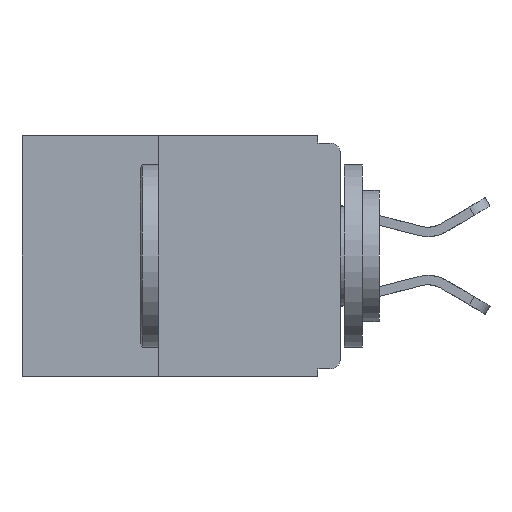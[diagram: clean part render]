
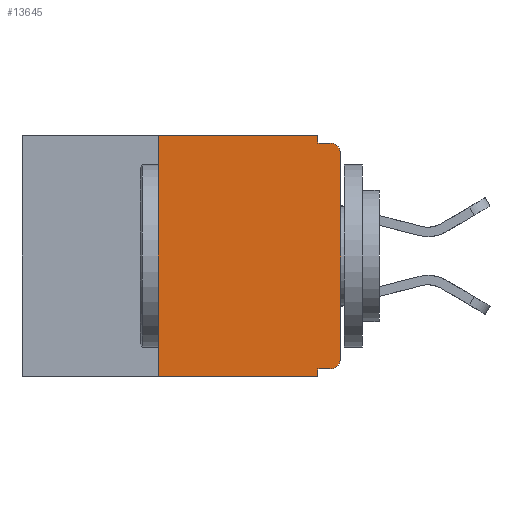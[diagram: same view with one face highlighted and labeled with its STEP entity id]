
A CAD part, left-side view. The second image highlights one B-rep face of the part: STEP entity #13645.
In plain terms, the highlighted planar face has unit normal (-1, 0, 0).
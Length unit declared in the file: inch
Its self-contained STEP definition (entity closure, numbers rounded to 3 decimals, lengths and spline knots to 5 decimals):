
#444 = EDGE_CURVE ( 'NONE', #15665, #19571, #15743, .T. ) ;
#541 = EDGE_CURVE ( 'NONE', #19571, #7961, #1320, .T. ) ;
#858 = CARTESIAN_POINT ( 'NONE',  ( 0., 0., 0. ) ) ;
#886 = LINE ( 'NONE', #4013, #8792 ) ;
#1320 = LINE ( 'NONE', #17184, #17396 ) ;
#1371 = ORIENTED_EDGE ( 'NONE', *, *, #14085, .F. ) ;
#1506 = VECTOR ( 'NONE', #18126, 39.37008 ) ;
#1526 = ORIENTED_EDGE ( 'NONE', *, *, #541, .F. ) ;
#1555 = DIRECTION ( 'NONE',  ( 0., 0., -1. ) ) ;
#1747 = ORIENTED_EDGE ( 'NONE', *, *, #4567, .T. ) ;
#1749 = ORIENTED_EDGE ( 'NONE', *, *, #18401, .T. ) ;
#2271 = DIRECTION ( 'NONE',  ( -1., 0., 0. ) ) ;
#2449 = DIRECTION ( 'NONE',  ( 0., 0., -1. ) ) ;
#2571 = ORIENTED_EDGE ( 'NONE', *, *, #444, .F. ) ;
#3269 = CARTESIAN_POINT ( 'NONE',  ( 0., 0.031, 0. ) ) ;
#3664 = ORIENTED_EDGE ( 'NONE', *, *, #14393, .F. ) ;
#4013 = CARTESIAN_POINT ( 'NONE',  ( 0., 0.031, -0.33 ) ) ;
#4156 = EDGE_CURVE ( 'NONE', #10617, #11605, #9327, .T. ) ;
#4250 = DIRECTION ( 'NONE',  ( 0., -1., 0. ) ) ;
#4461 = VECTOR ( 'NONE', #12520, 39.37008 ) ;
#4567 = EDGE_CURVE ( 'NONE', #10539, #11439, #19518, .T. ) ;
#4672 = CARTESIAN_POINT ( 'NONE',  ( 0., 0.437, 0. ) ) ;
#4849 = DIRECTION ( 'NONE',  ( 0., 1., 0. ) ) ;
#5137 = VECTOR ( 'NONE', #11499, 39.37008 ) ;
#5409 = VECTOR ( 'NONE', #5617, 39.37008 ) ;
#5617 = DIRECTION ( 'NONE',  ( 0., 0., 1. ) ) ;
#5686 = CARTESIAN_POINT ( 'NONE',  ( 0., 0.437, 0. ) ) ;
#6253 = PLANE ( 'NONE',  #17748 ) ;
#6375 = CARTESIAN_POINT ( 'NONE',  ( 0., 0.015, -0.32 ) ) ;
#6379 = ORIENTED_EDGE ( 'NONE', *, *, #7638, .T. ) ;
#6568 = CARTESIAN_POINT ( 'NONE',  ( 0., 0.25, -0.33 ) ) ;
#6708 = CARTESIAN_POINT ( 'NONE',  ( 0., 0.031, -0.33 ) ) ;
#6835 = EDGE_CURVE ( 'NONE', #10617, #7065, #15927, .T. ) ;
#6854 = ORIENTED_EDGE ( 'NONE', *, *, #4156, .F. ) ;
#6856 = EDGE_LOOP ( 'NONE', ( #6379, #1749, #1526, #2571, #1371, #6854, #17274, #17053, #3664, #1747 ) ) ;
#7065 = VERTEX_POINT ( 'NONE', #6708 ) ;
#7445 = CARTESIAN_POINT ( 'NONE',  ( 0., 0.25, 0. ) ) ;
#7638 = EDGE_CURVE ( 'NONE', #11439, #8525, #9589, .T. ) ;
#7961 = VERTEX_POINT ( 'NONE', #15674 ) ;
#8308 = VERTEX_POINT ( 'NONE', #17842 ) ;
#8525 = VERTEX_POINT ( 'NONE', #12263 ) ;
#8621 = CARTESIAN_POINT ( 'NONE',  ( 0., 0., -0.305 ) ) ;
#8653 = VECTOR ( 'NONE', #4849, 39.37008 ) ;
#8792 = VECTOR ( 'NONE', #2449, 39.37008 ) ;
#9327 = LINE ( 'NONE', #11340, #5137 ) ;
#9476 = EDGE_CURVE ( 'NONE', #8308, #7065, #886, .T. ) ;
#9589 = LINE ( 'NONE', #858, #5409 ) ;
#9760 = DIRECTION ( 'NONE',  ( 0., 0., -1. ) ) ;
#10539 = VERTEX_POINT ( 'NONE', #6375 ) ;
#10617 = VERTEX_POINT ( 'NONE', #6568 ) ;
#10971 = DIRECTION ( 'NONE',  ( 1., 0., 0. ) ) ;
#11340 = CARTESIAN_POINT ( 'NONE',  ( 0., 0.25, -0.33 ) ) ;
#11436 = CARTESIAN_POINT ( 'NONE',  ( 0., 0.031, 0. ) ) ;
#11439 = VERTEX_POINT ( 'NONE', #8621 ) ;
#11499 = DIRECTION ( 'NONE',  ( 0., 0., 1. ) ) ;
#11605 = VERTEX_POINT ( 'NONE', #7445 ) ;
#11636 = CARTESIAN_POINT ( 'NONE',  ( 0., 0.015, -0.025 ) ) ;
#12108 = VECTOR ( 'NONE', #9760, 39.37008 ) ;
#12263 = CARTESIAN_POINT ( 'NONE',  ( 0., 0., -0.025 ) ) ;
#12520 = DIRECTION ( 'NONE',  ( 0., -1., 0. ) ) ;
#12640 = CARTESIAN_POINT ( 'NONE',  ( 0., 0.437, -0.33 ) ) ;
#13180 = DIRECTION ( 'NONE',  ( 0., 0., -1. ) ) ;
#13354 = AXIS2_PLACEMENT_3D ( 'NONE', #19183, #18585, #18454 ) ;
#13510 = FACE_OUTER_BOUND ( 'NONE', #6856, .T. ) ;
#13645 = ADVANCED_FACE ( 'NONE', ( #13510 ), #6253, .F. ) ;
#13967 = LINE ( 'NONE', #5686, #1506 ) ;
#14085 = EDGE_CURVE ( 'NONE', #11605, #15665, #13967, .T. ) ;
#14163 = CARTESIAN_POINT ( 'NONE',  ( 0., 0., -0.32 ) ) ;
#14218 = CIRCLE ( 'NONE', #16807, 0.015 ) ;
#14393 = EDGE_CURVE ( 'NONE', #10539, #8308, #17785, .T. ) ;
#15233 = CARTESIAN_POINT ( 'NONE',  ( 0., 0.031, -0.01 ) ) ;
#15665 = VERTEX_POINT ( 'NONE', #3269 ) ;
#15674 = CARTESIAN_POINT ( 'NONE',  ( 0., 0.015, -0.01 ) ) ;
#15743 = LINE ( 'NONE', #11436, #12108 ) ;
#15927 = LINE ( 'NONE', #12640, #4461 ) ;
#16807 = AXIS2_PLACEMENT_3D ( 'NONE', #11636, #2271, #13180 ) ;
#17053 = ORIENTED_EDGE ( 'NONE', *, *, #9476, .F. ) ;
#17184 = CARTESIAN_POINT ( 'NONE',  ( 0., 0., -0.01 ) ) ;
#17274 = ORIENTED_EDGE ( 'NONE', *, *, #6835, .T. ) ;
#17396 = VECTOR ( 'NONE', #4250, 39.37008 ) ;
#17748 = AXIS2_PLACEMENT_3D ( 'NONE', #4672, #10971, #1555 ) ;
#17785 = LINE ( 'NONE', #14163, #8653 ) ;
#17842 = CARTESIAN_POINT ( 'NONE',  ( 0., 0.031, -0.32 ) ) ;
#18126 = DIRECTION ( 'NONE',  ( 0., -1., 0. ) ) ;
#18401 = EDGE_CURVE ( 'NONE', #8525, #7961, #14218, .T. ) ;
#18454 = DIRECTION ( 'NONE',  ( 0., 0., -1. ) ) ;
#18585 = DIRECTION ( 'NONE',  ( -1., 0., 0. ) ) ;
#19183 = CARTESIAN_POINT ( 'NONE',  ( 0., 0.015, -0.305 ) ) ;
#19518 = CIRCLE ( 'NONE', #13354, 0.015 ) ;
#19571 = VERTEX_POINT ( 'NONE', #15233 ) ;
